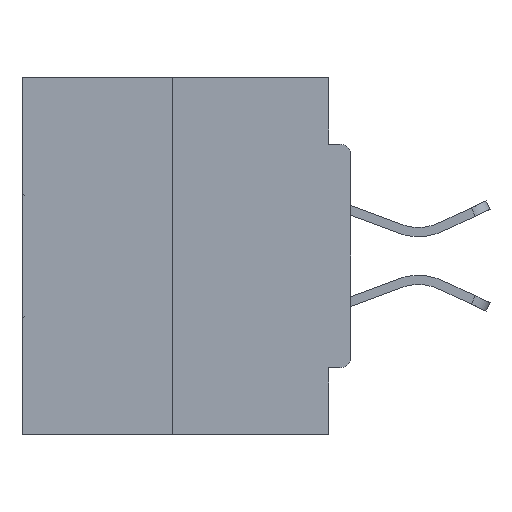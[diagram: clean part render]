
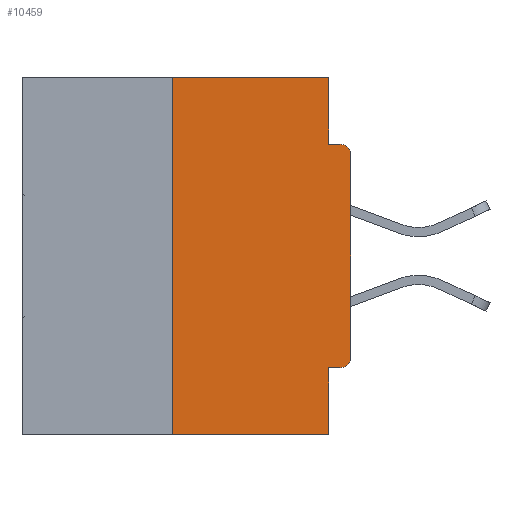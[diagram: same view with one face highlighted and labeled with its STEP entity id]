
A CAD part, left-side view. The second image highlights one B-rep face of the part: STEP entity #10459.
In plain terms, the highlighted planar face has unit normal (-1, 0, 0).
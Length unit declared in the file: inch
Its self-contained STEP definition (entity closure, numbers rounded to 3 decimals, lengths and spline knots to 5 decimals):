
#923 = ORIENTED_EDGE ( 'NONE', *, *, #24541, .F. ) ;
#966 = VECTOR ( 'NONE', #5476, 39.37008 ) ;
#1453 = EDGE_CURVE ( 'NONE', #8159, #26542, #34345, .T. ) ;
#1664 = DIRECTION ( 'NONE',  ( 0., 0., 1. ) ) ;
#1718 = DIRECTION ( 'NONE',  ( 0., -1., 0. ) ) ;
#1862 = LINE ( 'NONE', #23819, #17339 ) ;
#2069 = ORIENTED_EDGE ( 'NONE', *, *, #28446, .F. ) ;
#2127 = CARTESIAN_POINT ( 'NONE',  ( 0., 0.031, 0. ) ) ;
#2437 = VECTOR ( 'NONE', #1664, 39.37008 ) ;
#3248 = LINE ( 'NONE', #35440, #27624 ) ;
#3459 = LINE ( 'NONE', #14007, #27494 ) ;
#3641 = VECTOR ( 'NONE', #14210, 39.37008 ) ;
#4349 = AXIS2_PLACEMENT_3D ( 'NONE', #30601, #39840, #33537 ) ;
#5476 = DIRECTION ( 'NONE',  ( 0., 0., -1. ) ) ;
#5492 = VERTEX_POINT ( 'NONE', #34933 ) ;
#5963 = DIRECTION ( 'NONE',  ( 0., -1., 0. ) ) ;
#6819 = VERTEX_POINT ( 'NONE', #9462 ) ;
#7189 = CARTESIAN_POINT ( 'NONE',  ( 0., 0.25, 0. ) ) ;
#8159 = VERTEX_POINT ( 'NONE', #18827 ) ;
#8371 = AXIS2_PLACEMENT_3D ( 'NONE', #36489, #13849, #26602 ) ;
#9462 = CARTESIAN_POINT ( 'NONE',  ( 0., 0.015, -0.4065 ) ) ;
#9667 = EDGE_CURVE ( 'NONE', #20429, #5492, #20289, .T. ) ;
#9848 = ORIENTED_EDGE ( 'NONE', *, *, #12181, .T. ) ;
#10134 = ORIENTED_EDGE ( 'NONE', *, *, #17822, .T. ) ;
#10459 = ADVANCED_FACE ( 'NONE', ( #36895 ), #11360, .F. ) ;
#10502 = EDGE_CURVE ( 'NONE', #6819, #37083, #40457, .T. ) ;
#11360 = PLANE ( 'NONE',  #4349 ) ;
#11755 = VERTEX_POINT ( 'NONE', #40811 ) ;
#12181 = EDGE_CURVE ( 'NONE', #37083, #40385, #1862, .T. ) ;
#12562 = ORIENTED_EDGE ( 'NONE', *, *, #10502, .T. ) ;
#12875 = EDGE_CURVE ( 'NONE', #40385, #11755, #33463, .T. ) ;
#13763 = LINE ( 'NONE', #20643, #2437 ) ;
#13849 = DIRECTION ( 'NONE',  ( -1., 0., 0. ) ) ;
#14007 = CARTESIAN_POINT ( 'NONE',  ( 0., 0.46, 0. ) ) ;
#14210 = DIRECTION ( 'NONE',  ( 0., 0., -1. ) ) ;
#15344 = LINE ( 'NONE', #24559, #33953 ) ;
#15778 = DIRECTION ( 'NONE',  ( 0., -1., 0. ) ) ;
#16090 = EDGE_CURVE ( 'NONE', #19749, #8159, #3459, .T. ) ;
#17054 = CARTESIAN_POINT ( 'NONE',  ( 0., 0., -0.3915 ) ) ;
#17226 = VERTEX_POINT ( 'NONE', #30511 ) ;
#17339 = VECTOR ( 'NONE', #33447, 39.37008 ) ;
#17748 = ORIENTED_EDGE ( 'NONE', *, *, #1453, .F. ) ;
#17822 = EDGE_CURVE ( 'NONE', #17226, #5492, #3248, .T. ) ;
#18502 = DIRECTION ( 'NONE',  ( 0., 1., 0. ) ) ;
#18827 = CARTESIAN_POINT ( 'NONE',  ( 0., 0.031, 0. ) ) ;
#19749 = VERTEX_POINT ( 'NONE', #7189 ) ;
#19867 = CARTESIAN_POINT ( 'NONE',  ( 0., 0.031, -0.0935 ) ) ;
#20146 = ORIENTED_EDGE ( 'NONE', *, *, #16090, .F. ) ;
#20289 = LINE ( 'NONE', #29730, #3641 ) ;
#20429 = VERTEX_POINT ( 'NONE', #25032 ) ;
#20643 = CARTESIAN_POINT ( 'NONE',  ( 0., 0.25, 0. ) ) ;
#21665 = LINE ( 'NONE', #31292, #33449 ) ;
#22749 = EDGE_LOOP ( 'NONE', ( #20146, #39244, #10134, #35304, #2069, #12562, #9848, #25891, #923, #17748 ) ) ;
#23819 = CARTESIAN_POINT ( 'NONE',  ( 0., 0., 0. ) ) ;
#24541 = EDGE_CURVE ( 'NONE', #26542, #11755, #15344, .T. ) ;
#24559 = CARTESIAN_POINT ( 'NONE',  ( 0., 0., -0.0935 ) ) ;
#24760 = AXIS2_PLACEMENT_3D ( 'NONE', #28986, #32736, #36080 ) ;
#25032 = CARTESIAN_POINT ( 'NONE',  ( 0., 0.031, -0.4065 ) ) ;
#25891 = ORIENTED_EDGE ( 'NONE', *, *, #12875, .T. ) ;
#26331 = CARTESIAN_POINT ( 'NONE',  ( 0., 0., -0.1085 ) ) ;
#26542 = VERTEX_POINT ( 'NONE', #19867 ) ;
#26602 = DIRECTION ( 'NONE',  ( 0., 0., -1. ) ) ;
#27494 = VECTOR ( 'NONE', #1718, 39.37008 ) ;
#27624 = VECTOR ( 'NONE', #15778, 39.37008 ) ;
#28446 = EDGE_CURVE ( 'NONE', #6819, #20429, #21665, .T. ) ;
#28986 = CARTESIAN_POINT ( 'NONE',  ( 0., 0.015, -0.1085 ) ) ;
#29730 = CARTESIAN_POINT ( 'NONE',  ( 0., 0.031, -0.5 ) ) ;
#30511 = CARTESIAN_POINT ( 'NONE',  ( 0., 0.25, -0.5 ) ) ;
#30601 = CARTESIAN_POINT ( 'NONE',  ( 0., 0.46, 0. ) ) ;
#31292 = CARTESIAN_POINT ( 'NONE',  ( 0., 0., -0.4065 ) ) ;
#32736 = DIRECTION ( 'NONE',  ( -1., 0., 0. ) ) ;
#33447 = DIRECTION ( 'NONE',  ( 0., 0., 1. ) ) ;
#33449 = VECTOR ( 'NONE', #18502, 39.37008 ) ;
#33463 = CIRCLE ( 'NONE', #24760, 0.015 ) ;
#33537 = DIRECTION ( 'NONE',  ( 0., 0., -1. ) ) ;
#33953 = VECTOR ( 'NONE', #5963, 39.37008 ) ;
#34345 = LINE ( 'NONE', #2127, #966 ) ;
#34933 = CARTESIAN_POINT ( 'NONE',  ( 0., 0.031, -0.5 ) ) ;
#35304 = ORIENTED_EDGE ( 'NONE', *, *, #9667, .F. ) ;
#35440 = CARTESIAN_POINT ( 'NONE',  ( 0., 0.46, -0.5 ) ) ;
#35537 = EDGE_CURVE ( 'NONE', #17226, #19749, #13763, .T. ) ;
#36080 = DIRECTION ( 'NONE',  ( 0., 0., -1. ) ) ;
#36489 = CARTESIAN_POINT ( 'NONE',  ( 0., 0.015, -0.3915 ) ) ;
#36895 = FACE_OUTER_BOUND ( 'NONE', #22749, .T. ) ;
#37083 = VERTEX_POINT ( 'NONE', #17054 ) ;
#39244 = ORIENTED_EDGE ( 'NONE', *, *, #35537, .F. ) ;
#39840 = DIRECTION ( 'NONE',  ( 1., 0., 0. ) ) ;
#40385 = VERTEX_POINT ( 'NONE', #26331 ) ;
#40457 = CIRCLE ( 'NONE', #8371, 0.015 ) ;
#40811 = CARTESIAN_POINT ( 'NONE',  ( 0., 0.015, -0.0935 ) ) ;
